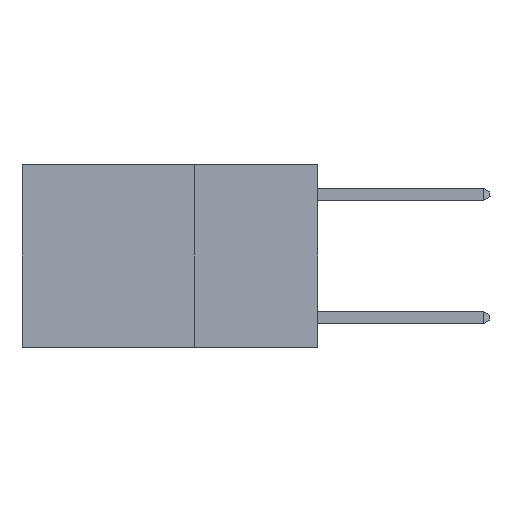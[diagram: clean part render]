
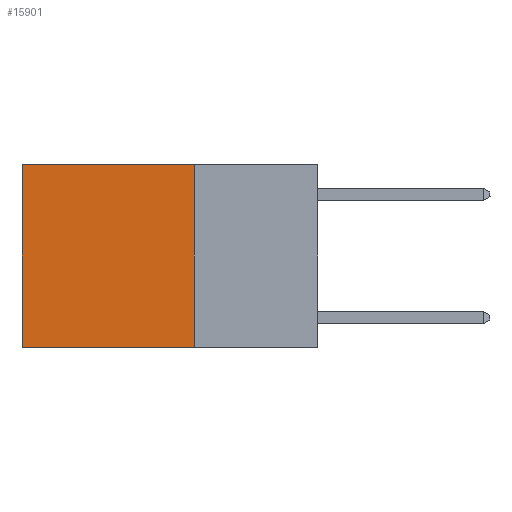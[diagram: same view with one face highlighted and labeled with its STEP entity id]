
A CAD part, left-side view. The second image highlights one B-rep face of the part: STEP entity #15901.
In plain terms, the highlighted planar face has unit normal (-1, 0, 0).
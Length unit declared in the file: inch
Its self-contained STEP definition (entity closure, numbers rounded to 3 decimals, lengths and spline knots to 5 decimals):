
#314 = VECTOR ( 'NONE', #21987, 39.37008 ) ;
#675 = CARTESIAN_POINT ( 'NONE',  ( 0.2625, 0.25, 0. ) ) ;
#716 = VERTEX_POINT ( 'NONE', #4460 ) ;
#1367 = LINE ( 'NONE', #10169, #14680 ) ;
#2390 = VERTEX_POINT ( 'NONE', #8792 ) ;
#2860 = LINE ( 'NONE', #7054, #21372 ) ;
#3457 = CARTESIAN_POINT ( 'NONE',  ( 0.2625, 0.6, 0. ) ) ;
#4460 = CARTESIAN_POINT ( 'NONE',  ( 0.2625, 0.6, -0.37 ) ) ;
#4805 = VECTOR ( 'NONE', #12205, 39.37008 ) ;
#6143 = LINE ( 'NONE', #675, #314 ) ;
#6371 = ORIENTED_EDGE ( 'NONE', *, *, #20750, .F. ) ;
#6485 = EDGE_LOOP ( 'NONE', ( #9938, #6371, #17352, #9366 ) ) ;
#7054 = CARTESIAN_POINT ( 'NONE',  ( 0.2625, 0.25, -0.37 ) ) ;
#7333 = LINE ( 'NONE', #3457, #4805 ) ;
#8026 = DIRECTION ( 'NONE',  ( 1., 0., 0. ) ) ;
#8104 = DIRECTION ( 'NONE',  ( 0., 0., -1. ) ) ;
#8123 = CARTESIAN_POINT ( 'NONE',  ( 0.2625, 0.6, 0. ) ) ;
#8792 = CARTESIAN_POINT ( 'NONE',  ( 0.2625, 0.25, -0.37 ) ) ;
#9366 = ORIENTED_EDGE ( 'NONE', *, *, #14619, .T. ) ;
#9380 = PLANE ( 'NONE',  #19006 ) ;
#9938 = ORIENTED_EDGE ( 'NONE', *, *, #18679, .T. ) ;
#10169 = CARTESIAN_POINT ( 'NONE',  ( 0.2625, 0.25, 0. ) ) ;
#12205 = DIRECTION ( 'NONE',  ( 0., 0., -1. ) ) ;
#12758 = VERTEX_POINT ( 'NONE', #21572 ) ;
#13333 = EDGE_CURVE ( 'NONE', #12758, #2390, #6143, .T. ) ;
#13426 = CARTESIAN_POINT ( 'NONE',  ( 0.2625, 0.25, 0. ) ) ;
#13690 = DIRECTION ( 'NONE',  ( 0., 1., 0. ) ) ;
#14619 = EDGE_CURVE ( 'NONE', #12758, #15269, #1367, .T. ) ;
#14680 = VECTOR ( 'NONE', #13690, 39.37008 ) ;
#15269 = VERTEX_POINT ( 'NONE', #8123 ) ;
#15901 = ADVANCED_FACE ( 'NONE', ( #20446 ), #9380, .F. ) ;
#17352 = ORIENTED_EDGE ( 'NONE', *, *, #13333, .F. ) ;
#17657 = DIRECTION ( 'NONE',  ( 0., 1., 0. ) ) ;
#18679 = EDGE_CURVE ( 'NONE', #15269, #716, #7333, .T. ) ;
#19006 = AXIS2_PLACEMENT_3D ( 'NONE', #13426, #8026, #8104 ) ;
#20446 = FACE_OUTER_BOUND ( 'NONE', #6485, .T. ) ;
#20750 = EDGE_CURVE ( 'NONE', #2390, #716, #2860, .T. ) ;
#21372 = VECTOR ( 'NONE', #17657, 39.37008 ) ;
#21572 = CARTESIAN_POINT ( 'NONE',  ( 0.2625, 0.25, 0. ) ) ;
#21987 = DIRECTION ( 'NONE',  ( 0., 0., -1. ) ) ;
